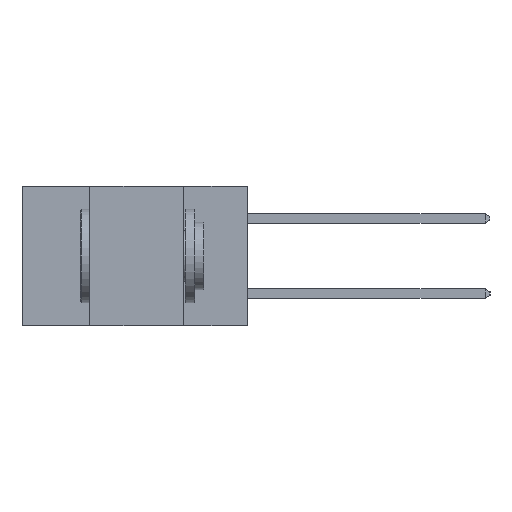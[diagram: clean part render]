
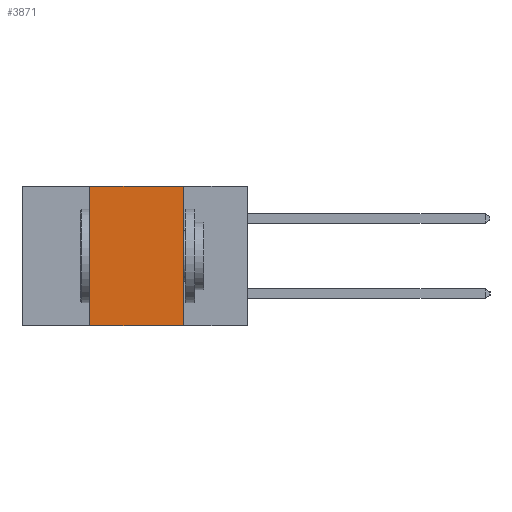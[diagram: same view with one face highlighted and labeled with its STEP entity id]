
A CAD part, left-side view. The second image highlights one B-rep face of the part: STEP entity #3871.
In plain terms, the highlighted planar face has unit normal (-1, 0, 0).
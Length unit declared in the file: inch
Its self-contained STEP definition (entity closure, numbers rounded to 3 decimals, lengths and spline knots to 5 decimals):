
#63 = CARTESIAN_POINT ( 'NONE',  ( 0., 0.17, -0.37 ) ) ;
#238 = VECTOR ( 'NONE', #7815, 39.37008 ) ;
#361 = CARTESIAN_POINT ( 'NONE',  ( 0., 0.17, 0. ) ) ;
#993 = CARTESIAN_POINT ( 'NONE',  ( 0., 0.42, 0. ) ) ;
#1030 = LINE ( 'NONE', #7589, #5040 ) ;
#1069 = VERTEX_POINT ( 'NONE', #63 ) ;
#1116 = CARTESIAN_POINT ( 'NONE',  ( 0., 0.6, 0. ) ) ;
#1164 = FACE_OUTER_BOUND ( 'NONE', #5677, .T. ) ;
#1450 = DIRECTION ( 'NONE',  ( 0., 0., -1. ) ) ;
#1498 = DIRECTION ( 'NONE',  ( 1., 0., 0. ) ) ;
#1607 = PLANE ( 'NONE',  #5980 ) ;
#2050 = DIRECTION ( 'NONE',  ( 0., -1., 0. ) ) ;
#3266 = VERTEX_POINT ( 'NONE', #993 ) ;
#3428 = ORIENTED_EDGE ( 'NONE', *, *, #4134, .F. ) ;
#3556 = EDGE_CURVE ( 'NONE', #4069, #1069, #6326, .T. ) ;
#3660 = VECTOR ( 'NONE', #2050, 39.37008 ) ;
#3871 = ADVANCED_FACE ( 'NONE', ( #1164 ), #1607, .F. ) ;
#3899 = LINE ( 'NONE', #5314, #3660 ) ;
#4069 = VERTEX_POINT ( 'NONE', #8201 ) ;
#4134 = EDGE_CURVE ( 'NONE', #4545, #1069, #1030, .T. ) ;
#4545 = VERTEX_POINT ( 'NONE', #361 ) ;
#5040 = VECTOR ( 'NONE', #7497, 39.37008 ) ;
#5314 = CARTESIAN_POINT ( 'NONE',  ( 0., 0.6, 0. ) ) ;
#5389 = EDGE_CURVE ( 'NONE', #4069, #3266, #8078, .T. ) ;
#5677 = EDGE_LOOP ( 'NONE', ( #3428, #6138, #6705, #9038 ) ) ;
#5833 = DIRECTION ( 'NONE',  ( 0., -1., 0. ) ) ;
#5923 = CARTESIAN_POINT ( 'NONE',  ( 0., 0.6, -0.37 ) ) ;
#5980 = AXIS2_PLACEMENT_3D ( 'NONE', #1116, #1498, #1450 ) ;
#6138 = ORIENTED_EDGE ( 'NONE', *, *, #9098, .F. ) ;
#6326 = LINE ( 'NONE', #5923, #10282 ) ;
#6705 = ORIENTED_EDGE ( 'NONE', *, *, #5389, .F. ) ;
#7497 = DIRECTION ( 'NONE',  ( 0., 0., -1. ) ) ;
#7589 = CARTESIAN_POINT ( 'NONE',  ( 0., 0.17, -0.37 ) ) ;
#7750 = CARTESIAN_POINT ( 'NONE',  ( 0., 0.42, -0.37 ) ) ;
#7815 = DIRECTION ( 'NONE',  ( 0., 0., 1. ) ) ;
#8078 = LINE ( 'NONE', #7750, #238 ) ;
#8201 = CARTESIAN_POINT ( 'NONE',  ( 0., 0.42, -0.37 ) ) ;
#9038 = ORIENTED_EDGE ( 'NONE', *, *, #3556, .T. ) ;
#9098 = EDGE_CURVE ( 'NONE', #3266, #4545, #3899, .T. ) ;
#10282 = VECTOR ( 'NONE', #5833, 39.37008 ) ;
